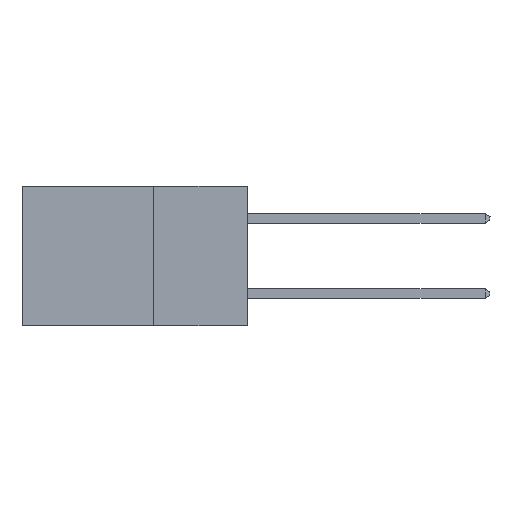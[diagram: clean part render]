
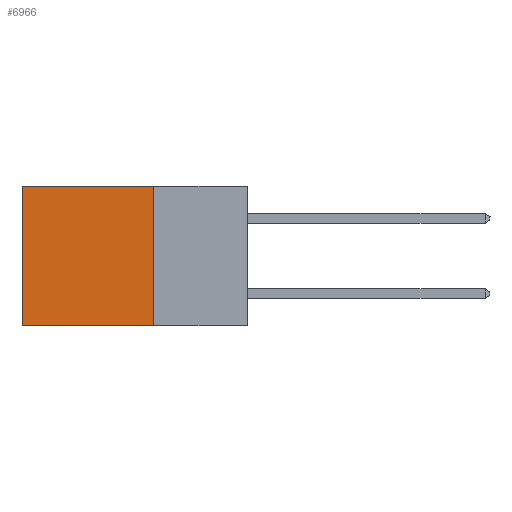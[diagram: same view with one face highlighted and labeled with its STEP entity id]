
A CAD part, left-side view. The second image highlights one B-rep face of the part: STEP entity #6966.
In plain terms, the highlighted planar face has unit normal (-1, 0, 0).
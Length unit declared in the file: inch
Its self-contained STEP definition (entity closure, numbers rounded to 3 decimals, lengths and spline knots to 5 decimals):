
#207 = VECTOR ( 'NONE', #13761, 39.37008 ) ;
#455 = FACE_OUTER_BOUND ( 'NONE', #5201, .T. ) ;
#487 = DIRECTION ( 'NONE',  ( 0., 0., -1. ) ) ;
#823 = VECTOR ( 'NONE', #487, 39.37008 ) ;
#1054 = CARTESIAN_POINT ( 'NONE',  ( 0.298, 0.25, -0.37 ) ) ;
#1102 = CARTESIAN_POINT ( 'NONE',  ( 0.298, 0.25, 0. ) ) ;
#1343 = CARTESIAN_POINT ( 'NONE',  ( 0.298, 0.25, 0. ) ) ;
#1881 = LINE ( 'NONE', #1343, #207 ) ;
#1932 = CARTESIAN_POINT ( 'NONE',  ( 0.298, 0.25, 0. ) ) ;
#2164 = VERTEX_POINT ( 'NONE', #9360 ) ;
#2231 = EDGE_CURVE ( 'NONE', #2164, #2982, #9707, .T. ) ;
#2295 = ORIENTED_EDGE ( 'NONE', *, *, #14617, .F. ) ;
#2982 = VERTEX_POINT ( 'NONE', #8692 ) ;
#3851 = PLANE ( 'NONE',  #15250 ) ;
#4745 = CARTESIAN_POINT ( 'NONE',  ( 0.298, 0.25, -0.37 ) ) ;
#5201 = EDGE_LOOP ( 'NONE', ( #9107, #2295, #10998, #15826 ) ) ;
#5498 = LINE ( 'NONE', #1054, #11508 ) ;
#6422 = LINE ( 'NONE', #1932, #14152 ) ;
#6759 = VERTEX_POINT ( 'NONE', #1102 ) ;
#6966 = ADVANCED_FACE ( 'NONE', ( #455 ), #3851, .F. ) ;
#8214 = VERTEX_POINT ( 'NONE', #4745 ) ;
#8341 = EDGE_CURVE ( 'NONE', #6759, #2164, #1881, .T. ) ;
#8692 = CARTESIAN_POINT ( 'NONE',  ( 0.298, 0.6, -0.37 ) ) ;
#9107 = ORIENTED_EDGE ( 'NONE', *, *, #2231, .T. ) ;
#9360 = CARTESIAN_POINT ( 'NONE',  ( 0.298, 0.6, 0. ) ) ;
#9612 = CARTESIAN_POINT ( 'NONE',  ( 0.298, 0.25, 0. ) ) ;
#9707 = LINE ( 'NONE', #11691, #823 ) ;
#9737 = DIRECTION ( 'NONE',  ( 0., 0., -1. ) ) ;
#10998 = ORIENTED_EDGE ( 'NONE', *, *, #12813, .F. ) ;
#11508 = VECTOR ( 'NONE', #17596, 39.37008 ) ;
#11691 = CARTESIAN_POINT ( 'NONE',  ( 0.298, 0.6, 0. ) ) ;
#12798 = DIRECTION ( 'NONE',  ( 0., 0., -1. ) ) ;
#12813 = EDGE_CURVE ( 'NONE', #6759, #8214, #6422, .T. ) ;
#13761 = DIRECTION ( 'NONE',  ( 0., 1., 0. ) ) ;
#14152 = VECTOR ( 'NONE', #12798, 39.37008 ) ;
#14617 = EDGE_CURVE ( 'NONE', #8214, #2982, #5498, .T. ) ;
#15250 = AXIS2_PLACEMENT_3D ( 'NONE', #9612, #16623, #9737 ) ;
#15826 = ORIENTED_EDGE ( 'NONE', *, *, #8341, .T. ) ;
#16623 = DIRECTION ( 'NONE',  ( 1., 0., 0. ) ) ;
#17596 = DIRECTION ( 'NONE',  ( 0., 1., 0. ) ) ;
